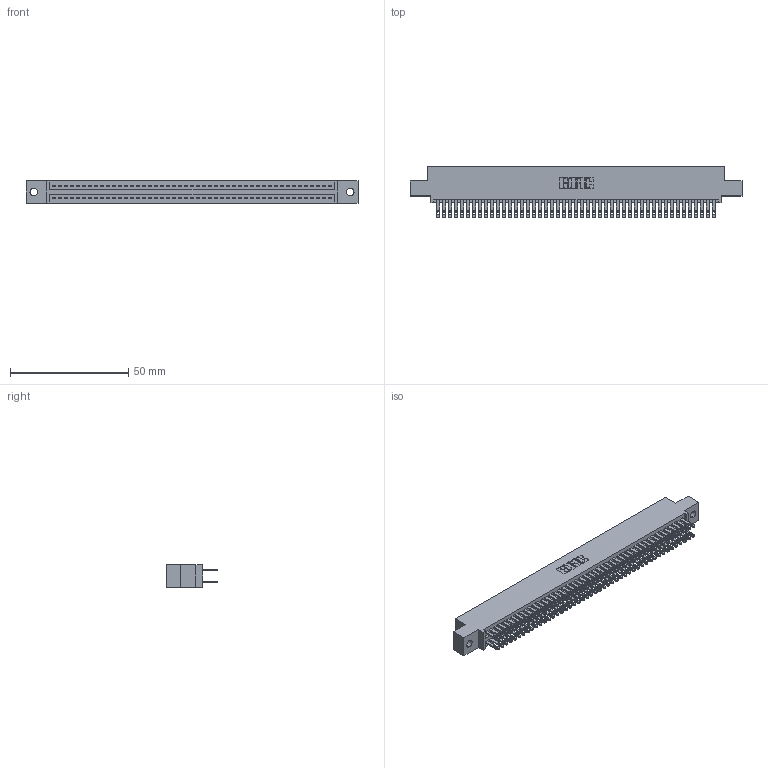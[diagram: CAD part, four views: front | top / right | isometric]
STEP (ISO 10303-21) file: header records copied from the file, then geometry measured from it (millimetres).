
FILE_DESCRIPTION (( 'STEP AP203' ), '1' );
FILE_NAME ('345-094-500-502.STEP', '2019-11-01T21:58:28', ( '' ), ( '' ), 'SwSTEP 2.0', 'SolidWorks 2016', '' );
FILE_SCHEMA (( 'CONFIG_CONTROL_DESIGN' ));
Length unit declared in the file: inch
Products named in the file (3): 345-094-500-502; 345 Part_0.110 Offset - 0.128 Dia; 345-292-001_345-293-100
Assembly tree (95 placements, depth 2):
  345-094-500-502
    345 Part_0.110 Offset - 0.128 Dia
    345-292-001_345-293-100  x94
Bounding box: 140.59 x 21.51 x 9.4 mm (x, y, z)
Volume: 13880.6 mm3; surface area: 21393.5 mm2
Topology: 95 solids, 95 shells, 4454 faces, 13607 edges, 9070 vertices
Faces by surface type: plane 2622, cylinder 1832
Entity records: 36269 total; most frequent: CARTESIAN_POINT 6076, ORIENTED_EDGE 6010, DIRECTION 5353, EDGE_CURVE 3005, LINE 2681, VECTOR 2681, VERTEX_POINT 2002, AXIS2_PLACEMENT_3D 1336
